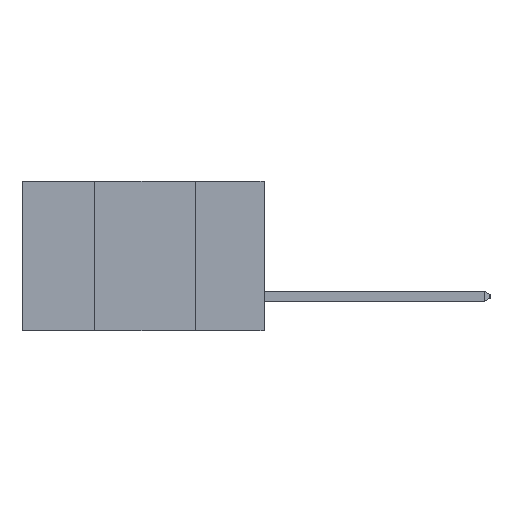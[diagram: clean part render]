
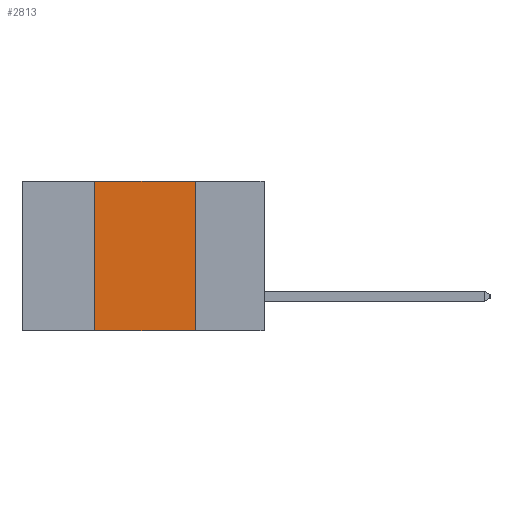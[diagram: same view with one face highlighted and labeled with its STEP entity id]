
A CAD part, left-side view. The second image highlights one B-rep face of the part: STEP entity #2813.
In plain terms, the highlighted planar face has unit normal (-1, 0, 0).
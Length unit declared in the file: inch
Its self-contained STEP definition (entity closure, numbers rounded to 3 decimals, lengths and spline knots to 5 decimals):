
#2690 = VERTEX_POINT ( 'NONE', #11363 ) ;
#2813 = ADVANCED_FACE ( 'NONE', ( #17187 ), #9767, .F. ) ;
#2983 = DIRECTION ( 'NONE',  ( 0., 0., 1. ) ) ;
#3306 = CARTESIAN_POINT ( 'NONE',  ( 0., 0.6, 0. ) ) ;
#5077 = LINE ( 'NONE', #17075, #9838 ) ;
#5140 = VERTEX_POINT ( 'NONE', #24952 ) ;
#5823 = EDGE_CURVE ( 'NONE', #2690, #10060, #18932, .T. ) ;
#8527 = EDGE_CURVE ( 'NONE', #2690, #5140, #5077, .T. ) ;
#8535 = DIRECTION ( 'NONE',  ( 0., -1., 0. ) ) ;
#8560 = LINE ( 'NONE', #21396, #18653 ) ;
#8601 = CARTESIAN_POINT ( 'NONE',  ( 0., 0.6, -0.37 ) ) ;
#9628 = AXIS2_PLACEMENT_3D ( 'NONE', #9736, #9702, #9697 ) ;
#9697 = DIRECTION ( 'NONE',  ( 0., 0., -1. ) ) ;
#9702 = DIRECTION ( 'NONE',  ( 1., 0., 0. ) ) ;
#9736 = CARTESIAN_POINT ( 'NONE',  ( 0., 0.6, 0. ) ) ;
#9767 = PLANE ( 'NONE',  #9628 ) ;
#9838 = VECTOR ( 'NONE', #2983, 39.37008 ) ;
#10060 = VERTEX_POINT ( 'NONE', #18100 ) ;
#11355 = CARTESIAN_POINT ( 'NONE',  ( 0., 0.17, 0. ) ) ;
#11363 = CARTESIAN_POINT ( 'NONE',  ( 0., 0.42, -0.37 ) ) ;
#11930 = LINE ( 'NONE', #3306, #12550 ) ;
#12550 = VECTOR ( 'NONE', #17400, 39.37008 ) ;
#13343 = ORIENTED_EDGE ( 'NONE', *, *, #5823, .T. ) ;
#13422 = DIRECTION ( 'NONE',  ( 0., 0., -1. ) ) ;
#15284 = EDGE_CURVE ( 'NONE', #5140, #17251, #11930, .T. ) ;
#17075 = CARTESIAN_POINT ( 'NONE',  ( 0., 0.42, -0.37 ) ) ;
#17187 = FACE_OUTER_BOUND ( 'NONE', #22945, .T. ) ;
#17251 = VERTEX_POINT ( 'NONE', #11355 ) ;
#17400 = DIRECTION ( 'NONE',  ( 0., -1., 0. ) ) ;
#17570 = ORIENTED_EDGE ( 'NONE', *, *, #8527, .F. ) ;
#17983 = EDGE_CURVE ( 'NONE', #17251, #10060, #8560, .T. ) ;
#18100 = CARTESIAN_POINT ( 'NONE',  ( 0., 0.17, -0.37 ) ) ;
#18310 = VECTOR ( 'NONE', #8535, 39.37008 ) ;
#18653 = VECTOR ( 'NONE', #13422, 39.37008 ) ;
#18932 = LINE ( 'NONE', #8601, #18310 ) ;
#21396 = CARTESIAN_POINT ( 'NONE',  ( 0., 0.17, -0.37 ) ) ;
#22059 = ORIENTED_EDGE ( 'NONE', *, *, #17983, .F. ) ;
#22945 = EDGE_LOOP ( 'NONE', ( #22059, #24490, #17570, #13343 ) ) ;
#24490 = ORIENTED_EDGE ( 'NONE', *, *, #15284, .F. ) ;
#24952 = CARTESIAN_POINT ( 'NONE',  ( 0., 0.42, 0. ) ) ;
